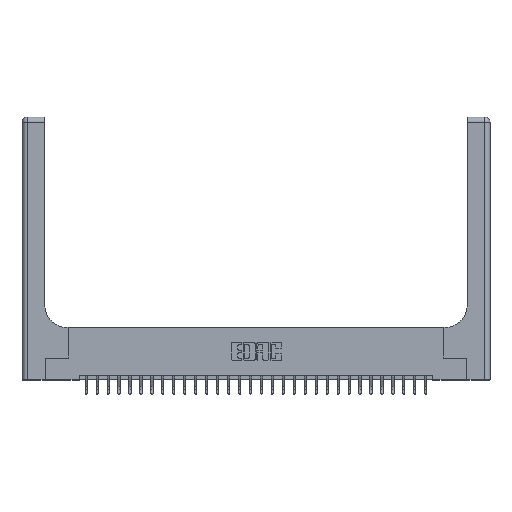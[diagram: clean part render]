
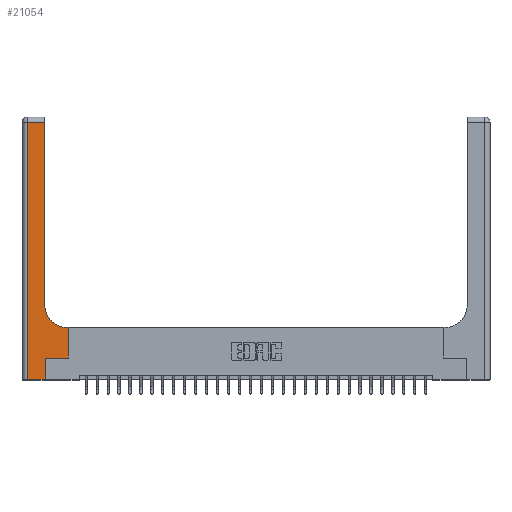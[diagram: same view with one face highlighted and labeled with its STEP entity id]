
A CAD part, top view. The second image highlights one B-rep face of the part: STEP entity #21054.
In plain terms, the highlighted planar face has unit normal (0, 0, 1).
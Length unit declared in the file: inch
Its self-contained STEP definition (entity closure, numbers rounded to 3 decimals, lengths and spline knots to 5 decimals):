
#32 = CARTESIAN_POINT ( 'NONE',  ( 0.06, 3., 0.37 ) ) ;
#35 = CARTESIAN_POINT ( 'NONE',  ( 0.528, 0.25, 0.37 ) ) ;
#41 = VECTOR ( 'NONE', #8477, 39.37008 ) ;
#71 = EDGE_LOOP ( 'NONE', ( #26118, #24265, #2680, #14399, #8236, #25777, #25832, #21047, #20861 ) ) ;
#269 = VERTEX_POINT ( 'NONE', #20532 ) ;
#533 = EDGE_CURVE ( 'NONE', #1671, #14499, #1143, .T. ) ;
#755 = VERTEX_POINT ( 'NONE', #21468 ) ;
#1143 = CIRCLE ( 'NONE', #14860, 0.25 ) ;
#1330 = VERTEX_POINT ( 'NONE', #13047 ) ;
#1671 = VERTEX_POINT ( 'NONE', #25113 ) ;
#2109 = CARTESIAN_POINT ( 'NONE',  ( 0.528, 0.25, 0.37 ) ) ;
#2609 = VECTOR ( 'NONE', #27385, 39.37008 ) ;
#2680 = ORIENTED_EDGE ( 'NONE', *, *, #9793, .T. ) ;
#3376 = DIRECTION ( 'NONE',  ( 0., 0., -1. ) ) ;
#3987 = DIRECTION ( 'NONE',  ( 1., 0., 0. ) ) ;
#4282 = DIRECTION ( 'NONE',  ( 0., -1., 0. ) ) ;
#4696 = LINE ( 'NONE', #35, #41 ) ;
#4852 = LINE ( 'NONE', #22397, #9475 ) ;
#5047 = DIRECTION ( 'NONE',  ( -1., 0., 0. ) ) ;
#5248 = DIRECTION ( 'NONE',  ( 1., 0., 0. ) ) ;
#5745 = LINE ( 'NONE', #32, #24816 ) ;
#7204 = CARTESIAN_POINT ( 'NONE',  ( 0.06, 2.94, 0.37 ) ) ;
#8236 = ORIENTED_EDGE ( 'NONE', *, *, #23329, .T. ) ;
#8477 = DIRECTION ( 'NONE',  ( 0., 1., 0. ) ) ;
#9475 = VECTOR ( 'NONE', #12294, 39.37008 ) ;
#9490 = VERTEX_POINT ( 'NONE', #19775 ) ;
#9793 = EDGE_CURVE ( 'NONE', #21437, #9490, #5745, .T. ) ;
#10913 = EDGE_CURVE ( 'NONE', #16658, #269, #4696, .T. ) ;
#11104 = CARTESIAN_POINT ( 'NONE',  ( 0., 3., 0.37 ) ) ;
#11312 = VECTOR ( 'NONE', #26229, 39.37008 ) ;
#11879 = CARTESIAN_POINT ( 'NONE',  ( 0.26, 0.85, 0.37 ) ) ;
#12294 = DIRECTION ( 'NONE',  ( -1., 0., 0. ) ) ;
#12579 = EDGE_CURVE ( 'NONE', #14499, #15299, #21937, .T. ) ;
#12685 = LINE ( 'NONE', #13631, #15364 ) ;
#13047 = CARTESIAN_POINT ( 'NONE',  ( 0.265, 0., 0.37 ) ) ;
#13631 = CARTESIAN_POINT ( 'NONE',  ( 0.265, 0.25, 0.37 ) ) ;
#13715 = DIRECTION ( 'NONE',  ( 1., 0., 0. ) ) ;
#14353 = EDGE_CURVE ( 'NONE', #755, #16658, #12685, .T. ) ;
#14399 = ORIENTED_EDGE ( 'NONE', *, *, #26082, .T. ) ;
#14499 = VERTEX_POINT ( 'NONE', #11879 ) ;
#14860 = AXIS2_PLACEMENT_3D ( 'NONE', #21135, #20764, #3987 ) ;
#15299 = VERTEX_POINT ( 'NONE', #15951 ) ;
#15364 = VECTOR ( 'NONE', #5248, 39.37008 ) ;
#15583 = CARTESIAN_POINT ( 'NONE',  ( 0., 0., 0.37 ) ) ;
#15951 = CARTESIAN_POINT ( 'NONE',  ( 0.26, 2.94, 0.37 ) ) ;
#16086 = EDGE_CURVE ( 'NONE', #269, #1671, #19290, .T. ) ;
#16533 = CARTESIAN_POINT ( 'NONE',  ( 0.26, 0.6, 0.37 ) ) ;
#16658 = VERTEX_POINT ( 'NONE', #2109 ) ;
#18653 = CARTESIAN_POINT ( 'NONE',  ( 0.265, 0., 0.37 ) ) ;
#18716 = DIRECTION ( 'NONE',  ( -1., 0., 0. ) ) ;
#18860 = VECTOR ( 'NONE', #13715, 39.37008 ) ;
#19290 = LINE ( 'NONE', #16533, #20289 ) ;
#19775 = CARTESIAN_POINT ( 'NONE',  ( 0.06, 0., 0.37 ) ) ;
#20289 = VECTOR ( 'NONE', #18716, 39.37008 ) ;
#20355 = LINE ( 'NONE', #18653, #11312 ) ;
#20462 = AXIS2_PLACEMENT_3D ( 'NONE', #11104, #3376, #5047 ) ;
#20532 = CARTESIAN_POINT ( 'NONE',  ( 0.528, 0.6, 0.37 ) ) ;
#20764 = DIRECTION ( 'NONE',  ( 0., 0., -1. ) ) ;
#20861 = ORIENTED_EDGE ( 'NONE', *, *, #533, .T. ) ;
#21047 = ORIENTED_EDGE ( 'NONE', *, *, #16086, .T. ) ;
#21054 = ADVANCED_FACE ( 'NONE', ( #22451 ), #21652, .F. ) ;
#21135 = CARTESIAN_POINT ( 'NONE',  ( 0.51, 0.85, 0.37 ) ) ;
#21437 = VERTEX_POINT ( 'NONE', #7204 ) ;
#21468 = CARTESIAN_POINT ( 'NONE',  ( 0.265, 0.25, 0.37 ) ) ;
#21652 = PLANE ( 'NONE',  #20462 ) ;
#21937 = LINE ( 'NONE', #27284, #2609 ) ;
#22397 = CARTESIAN_POINT ( 'NONE',  ( 0., 2.94, 0.37 ) ) ;
#22451 = FACE_OUTER_BOUND ( 'NONE', #71, .T. ) ;
#22504 = LINE ( 'NONE', #15583, #18860 ) ;
#23329 = EDGE_CURVE ( 'NONE', #1330, #755, #20355, .T. ) ;
#24265 = ORIENTED_EDGE ( 'NONE', *, *, #25800, .T. ) ;
#24816 = VECTOR ( 'NONE', #4282, 39.37008 ) ;
#25113 = CARTESIAN_POINT ( 'NONE',  ( 0.51, 0.6, 0.37 ) ) ;
#25777 = ORIENTED_EDGE ( 'NONE', *, *, #14353, .T. ) ;
#25800 = EDGE_CURVE ( 'NONE', #15299, #21437, #4852, .T. ) ;
#25832 = ORIENTED_EDGE ( 'NONE', *, *, #10913, .T. ) ;
#26082 = EDGE_CURVE ( 'NONE', #9490, #1330, #22504, .T. ) ;
#26118 = ORIENTED_EDGE ( 'NONE', *, *, #12579, .T. ) ;
#26229 = DIRECTION ( 'NONE',  ( 0., 1., 0. ) ) ;
#27284 = CARTESIAN_POINT ( 'NONE',  ( 0.26, 3., 0.37 ) ) ;
#27385 = DIRECTION ( 'NONE',  ( 0., 1., 0. ) ) ;
